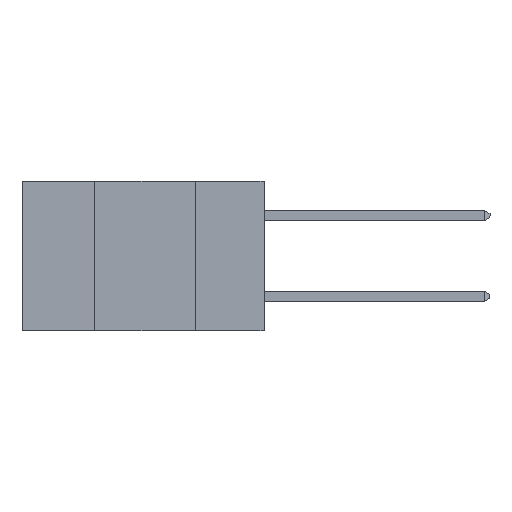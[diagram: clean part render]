
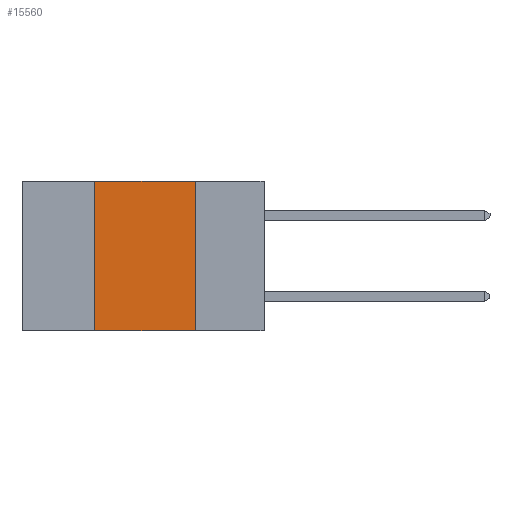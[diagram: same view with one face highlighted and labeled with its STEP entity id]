
A CAD part, left-side view. The second image highlights one B-rep face of the part: STEP entity #15560.
In plain terms, the highlighted planar face has unit normal (-1, 0, 0).
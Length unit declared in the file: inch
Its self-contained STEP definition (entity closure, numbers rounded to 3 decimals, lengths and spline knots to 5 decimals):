
#608 = DIRECTION ( 'NONE',  ( 1., 0., 0. ) ) ;
#773 = EDGE_CURVE ( 'NONE', #20691, #17641, #20590, .T. ) ;
#947 = CARTESIAN_POINT ( 'NONE',  ( 0., 0.42, 0. ) ) ;
#1820 = VECTOR ( 'NONE', #6299, 39.37008 ) ;
#2751 = ORIENTED_EDGE ( 'NONE', *, *, #11831, .F. ) ;
#2980 = ORIENTED_EDGE ( 'NONE', *, *, #10393, .F. ) ;
#3114 = ORIENTED_EDGE ( 'NONE', *, *, #7518, .F. ) ;
#3393 = ORIENTED_EDGE ( 'NONE', *, *, #773, .T. ) ;
#5079 = CARTESIAN_POINT ( 'NONE',  ( 0., 0.17, -0.37 ) ) ;
#5954 = CARTESIAN_POINT ( 'NONE',  ( 0., 0.17, 0. ) ) ;
#6217 = VECTOR ( 'NONE', #9549, 39.37008 ) ;
#6299 = DIRECTION ( 'NONE',  ( 0., -1., 0. ) ) ;
#6305 = CARTESIAN_POINT ( 'NONE',  ( 0., 0.6, -0.37 ) ) ;
#6732 = FACE_OUTER_BOUND ( 'NONE', #15194, .T. ) ;
#6806 = LINE ( 'NONE', #7731, #6217 ) ;
#7518 = EDGE_CURVE ( 'NONE', #20691, #14007, #15974, .T. ) ;
#7731 = CARTESIAN_POINT ( 'NONE',  ( 0., 0.6, 0. ) ) ;
#8105 = CARTESIAN_POINT ( 'NONE',  ( 0., 0.42, -0.37 ) ) ;
#9549 = DIRECTION ( 'NONE',  ( 0., -1., 0. ) ) ;
#10393 = EDGE_CURVE ( 'NONE', #14007, #13163, #6806, .T. ) ;
#10699 = VECTOR ( 'NONE', #18275, 39.37008 ) ;
#11831 = EDGE_CURVE ( 'NONE', #13163, #17641, #22935, .T. ) ;
#11899 = CARTESIAN_POINT ( 'NONE',  ( 0., 0.6, 0. ) ) ;
#13163 = VERTEX_POINT ( 'NONE', #21688 ) ;
#13631 = VECTOR ( 'NONE', #15086, 39.37008 ) ;
#13707 = DIRECTION ( 'NONE',  ( 0., 0., -1. ) ) ;
#14007 = VERTEX_POINT ( 'NONE', #947 ) ;
#15086 = DIRECTION ( 'NONE',  ( 0., 0., -1. ) ) ;
#15194 = EDGE_LOOP ( 'NONE', ( #2751, #2980, #3114, #3393 ) ) ;
#15560 = ADVANCED_FACE ( 'NONE', ( #6732 ), #18877, .F. ) ;
#15974 = LINE ( 'NONE', #23499, #10699 ) ;
#17641 = VERTEX_POINT ( 'NONE', #5079 ) ;
#18275 = DIRECTION ( 'NONE',  ( 0., 0., 1. ) ) ;
#18877 = PLANE ( 'NONE',  #22150 ) ;
#20590 = LINE ( 'NONE', #6305, #1820 ) ;
#20691 = VERTEX_POINT ( 'NONE', #8105 ) ;
#21688 = CARTESIAN_POINT ( 'NONE',  ( 0., 0.17, 0. ) ) ;
#22150 = AXIS2_PLACEMENT_3D ( 'NONE', #11899, #608, #13707 ) ;
#22935 = LINE ( 'NONE', #5954, #13631 ) ;
#23499 = CARTESIAN_POINT ( 'NONE',  ( 0., 0.42, 0. ) ) ;
